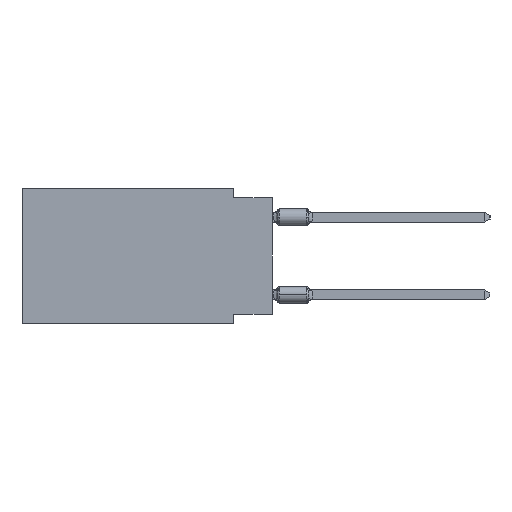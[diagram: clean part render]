
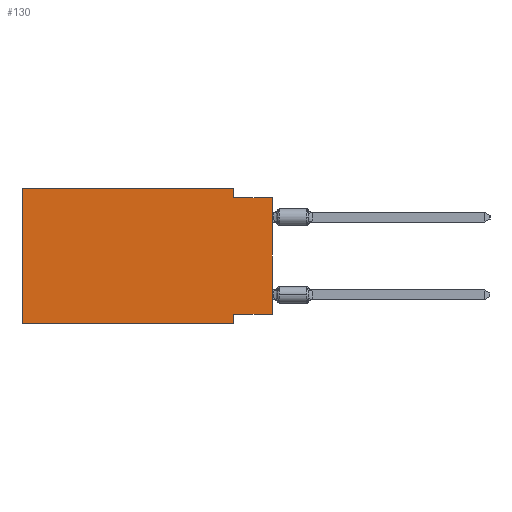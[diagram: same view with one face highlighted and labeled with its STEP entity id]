
A CAD part, left-side view. The second image highlights one B-rep face of the part: STEP entity #130.
In plain terms, the highlighted planar face has unit normal (-1, 0, 0).
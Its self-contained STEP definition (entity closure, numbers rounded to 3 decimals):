
#130 = ADVANCED_FACE ( 'NONE', ( #9887 ), #11543, .F. ) ;
#579 = CARTESIAN_POINT ( 'NONE',  ( 0., 0., -8.255 ) ) ;
#1662 = LINE ( 'NONE', #8956, #5114 ) ;
#1728 = VECTOR ( 'NONE', #18255, 1000. ) ;
#1947 = CARTESIAN_POINT ( 'NONE',  ( 0., 2.54, 0. ) ) ;
#1978 = VERTEX_POINT ( 'NONE', #12435 ) ;
#2434 = ORIENTED_EDGE ( 'NONE', *, *, #26765, .F. ) ;
#2762 = CARTESIAN_POINT ( 'NONE',  ( 0., 16.383, 0. ) ) ;
#3778 = CARTESIAN_POINT ( 'NONE',  ( 0., 0., -8.255 ) ) ;
#4386 = ORIENTED_EDGE ( 'NONE', *, *, #10269, .F. ) ;
#4413 = CARTESIAN_POINT ( 'NONE',  ( 0., 16.383, 0. ) ) ;
#4688 = VECTOR ( 'NONE', #19125, 1000. ) ;
#4762 = DIRECTION ( 'NONE',  ( 0., 0., 1. ) ) ;
#5114 = VECTOR ( 'NONE', #13128, 1000. ) ;
#5621 = ORIENTED_EDGE ( 'NONE', *, *, #12670, .T. ) ;
#6649 = LINE ( 'NONE', #4413, #1728 ) ;
#7000 = LINE ( 'NONE', #22773, #16857 ) ;
#7486 = ORIENTED_EDGE ( 'NONE', *, *, #12541, .F. ) ;
#7995 = CARTESIAN_POINT ( 'NONE',  ( 0., 0., -0.635 ) ) ;
#8488 = LINE ( 'NONE', #1947, #25843 ) ;
#8754 = EDGE_LOOP ( 'NONE', ( #5621, #12459, #7486, #2434, #28240, #15174, #19404, #4386 ) ) ;
#8956 = CARTESIAN_POINT ( 'NONE',  ( 0., 0., -0.635 ) ) ;
#9649 = CARTESIAN_POINT ( 'NONE',  ( 0., 16.383, 0. ) ) ;
#9887 = FACE_OUTER_BOUND ( 'NONE', #8754, .T. ) ;
#10092 = CARTESIAN_POINT ( 'NONE',  ( 0., 16.383, -8.89 ) ) ;
#10269 = EDGE_CURVE ( 'NONE', #21802, #19654, #28756, .T. ) ;
#10618 = CARTESIAN_POINT ( 'NONE',  ( 0., 2.54, 0. ) ) ;
#11048 = EDGE_CURVE ( 'NONE', #19282, #1978, #26014, .T. ) ;
#11219 = DIRECTION ( 'NONE',  ( 0., 0., -1. ) ) ;
#11543 = PLANE ( 'NONE',  #27789 ) ;
#12435 = CARTESIAN_POINT ( 'NONE',  ( 0., 2.54, -8.89 ) ) ;
#12459 = ORIENTED_EDGE ( 'NONE', *, *, #29273, .F. ) ;
#12541 = EDGE_CURVE ( 'NONE', #26269, #20147, #8488, .T. ) ;
#12631 = DIRECTION ( 'NONE',  ( 0., -1., 0. ) ) ;
#12670 = EDGE_CURVE ( 'NONE', #21802, #19630, #7000, .T. ) ;
#13128 = DIRECTION ( 'NONE',  ( 0., -1., 0. ) ) ;
#13742 = LINE ( 'NONE', #24603, #17930 ) ;
#15174 = ORIENTED_EDGE ( 'NONE', *, *, #11048, .T. ) ;
#15310 = CARTESIAN_POINT ( 'NONE',  ( 0., 16.383, -8.89 ) ) ;
#16693 = CARTESIAN_POINT ( 'NONE',  ( 0., 2.54, -0.635 ) ) ;
#16857 = VECTOR ( 'NONE', #4762, 1000. ) ;
#17930 = VECTOR ( 'NONE', #11219, 1000. ) ;
#18255 = DIRECTION ( 'NONE',  ( 0., 0., 1. ) ) ;
#18443 = LINE ( 'NONE', #9649, #19062 ) ;
#19062 = VECTOR ( 'NONE', #27211, 1000. ) ;
#19125 = DIRECTION ( 'NONE',  ( 0., 1., 0. ) ) ;
#19282 = VERTEX_POINT ( 'NONE', #15310 ) ;
#19404 = ORIENTED_EDGE ( 'NONE', *, *, #28851, .F. ) ;
#19630 = VERTEX_POINT ( 'NONE', #7995 ) ;
#19654 = VERTEX_POINT ( 'NONE', #21967 ) ;
#20147 = VERTEX_POINT ( 'NONE', #16693 ) ;
#21802 = VERTEX_POINT ( 'NONE', #579 ) ;
#21967 = CARTESIAN_POINT ( 'NONE',  ( 0., 2.54, -8.255 ) ) ;
#22773 = CARTESIAN_POINT ( 'NONE',  ( 0., 0., 0. ) ) ;
#23722 = VECTOR ( 'NONE', #12631, 1000. ) ;
#24603 = CARTESIAN_POINT ( 'NONE',  ( 0., 2.54, -8.89 ) ) ;
#24718 = VERTEX_POINT ( 'NONE', #27869 ) ;
#25218 = DIRECTION ( 'NONE',  ( 0., 0., -1. ) ) ;
#25843 = VECTOR ( 'NONE', #26935, 1000. ) ;
#26014 = LINE ( 'NONE', #10092, #23722 ) ;
#26269 = VERTEX_POINT ( 'NONE', #10618 ) ;
#26765 = EDGE_CURVE ( 'NONE', #24718, #26269, #18443, .T. ) ;
#26935 = DIRECTION ( 'NONE',  ( 0., 0., -1. ) ) ;
#27211 = DIRECTION ( 'NONE',  ( 0., -1., 0. ) ) ;
#27305 = DIRECTION ( 'NONE',  ( 1., 0., 0. ) ) ;
#27789 = AXIS2_PLACEMENT_3D ( 'NONE', #2762, #27305, #25218 ) ;
#27869 = CARTESIAN_POINT ( 'NONE',  ( 0., 16.383, 0. ) ) ;
#28240 = ORIENTED_EDGE ( 'NONE', *, *, #28484, .F. ) ;
#28484 = EDGE_CURVE ( 'NONE', #19282, #24718, #6649, .T. ) ;
#28756 = LINE ( 'NONE', #3778, #4688 ) ;
#28851 = EDGE_CURVE ( 'NONE', #19654, #1978, #13742, .T. ) ;
#29273 = EDGE_CURVE ( 'NONE', #20147, #19630, #1662, .T. ) ;
